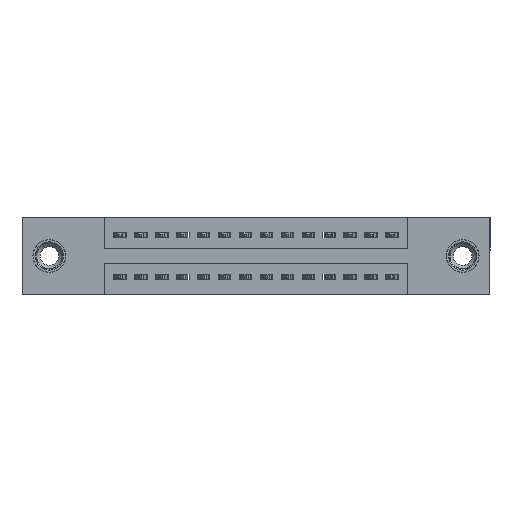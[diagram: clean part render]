
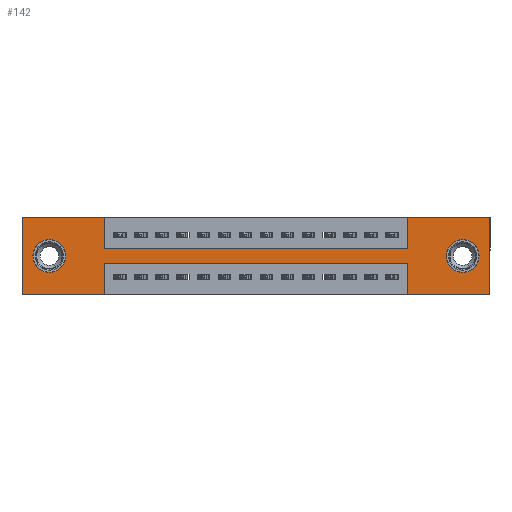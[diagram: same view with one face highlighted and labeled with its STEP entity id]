
A CAD part, front view. The second image highlights one B-rep face of the part: STEP entity #142.
In plain terms, the highlighted planar face has unit normal (0, -1, 0).
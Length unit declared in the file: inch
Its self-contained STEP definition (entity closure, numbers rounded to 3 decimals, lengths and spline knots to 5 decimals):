
#63 = VECTOR ( 'NONE', #2689, 39.37008 ) ;
#142 = ADVANCED_FACE ( 'NONE', ( #17013, #1408, #9060 ), #14671, .T. ) ;
#169 = VERTEX_POINT ( 'NONE', #14164 ) ;
#590 = CIRCLE ( 'NONE', #18414, 0.078 ) ;
#950 = CARTESIAN_POINT ( 'NONE',  ( 2.235, 0., 0. ) ) ;
#978 = CARTESIAN_POINT ( 'NONE',  ( 1.8425, 0., 0. ) ) ;
#983 = VERTEX_POINT ( 'NONE', #18829 ) ;
#1070 = CIRCLE ( 'NONE', #3841, 0.078 ) ;
#1088 = ORIENTED_EDGE ( 'NONE', *, *, #15698, .F. ) ;
#1398 = CARTESIAN_POINT ( 'NONE',  ( 2.105, 0., -0.107 ) ) ;
#1408 = FACE_BOUND ( 'NONE', #16963, .T. ) ;
#1886 = DIRECTION ( 'NONE',  ( 0., 0., -1. ) ) ;
#2145 = EDGE_CURVE ( 'NONE', #16153, #7513, #15894, .T. ) ;
#2438 = DIRECTION ( 'NONE',  ( 1., 0., 0. ) ) ;
#2542 = CARTESIAN_POINT ( 'NONE',  ( 2.105, 0., -0.185 ) ) ;
#2689 = DIRECTION ( 'NONE',  ( -1., 0., 0. ) ) ;
#2697 = VERTEX_POINT ( 'NONE', #13400 ) ;
#2744 = ORIENTED_EDGE ( 'NONE', *, *, #16561, .F. ) ;
#2795 = ORIENTED_EDGE ( 'NONE', *, *, #18884, .T. ) ;
#2824 = LINE ( 'NONE', #17985, #13924 ) ;
#2938 = EDGE_CURVE ( 'NONE', #16693, #10378, #7676, .T. ) ;
#3179 = ORIENTED_EDGE ( 'NONE', *, *, #10170, .F. ) ;
#3204 = LINE ( 'NONE', #4451, #18635 ) ;
#3341 = CARTESIAN_POINT ( 'NONE',  ( 1.8425, 0., -0.37 ) ) ;
#3640 = VECTOR ( 'NONE', #6353, 39.37008 ) ;
#3841 = AXIS2_PLACEMENT_3D ( 'NONE', #2542, #13101, #4074 ) ;
#3911 = CARTESIAN_POINT ( 'NONE',  ( 0.3925, 0., -0.15 ) ) ;
#4001 = ORIENTED_EDGE ( 'NONE', *, *, #4603, .T. ) ;
#4074 = DIRECTION ( 'NONE',  ( 0., 0., -1. ) ) ;
#4122 = LINE ( 'NONE', #4851, #3640 ) ;
#4193 = VERTEX_POINT ( 'NONE', #12833 ) ;
#4451 = CARTESIAN_POINT ( 'NONE',  ( 0., 0., 0. ) ) ;
#4603 = EDGE_CURVE ( 'NONE', #14933, #15991, #590, .T. ) ;
#4646 = ORIENTED_EDGE ( 'NONE', *, *, #14055, .T. ) ;
#4661 = VECTOR ( 'NONE', #6580, 39.37008 ) ;
#4756 = EDGE_CURVE ( 'NONE', #4193, #2697, #13933, .T. ) ;
#4851 = CARTESIAN_POINT ( 'NONE',  ( 0.3925, 0., -0.22 ) ) ;
#4906 = CARTESIAN_POINT ( 'NONE',  ( 1.8425, 0., -0.37 ) ) ;
#5013 = DIRECTION ( 'NONE',  ( 0., 1., 0. ) ) ;
#5074 = DIRECTION ( 'NONE',  ( 0., 0., -1. ) ) ;
#5104 = CARTESIAN_POINT ( 'NONE',  ( 0., 0., -0.37 ) ) ;
#5233 = LINE ( 'NONE', #8733, #63 ) ;
#5381 = DIRECTION ( 'NONE',  ( 0., 1., 0. ) ) ;
#5445 = DIRECTION ( 'NONE',  ( 0., 0., -1. ) ) ;
#5567 = DIRECTION ( 'NONE',  ( 0., -1., 0. ) ) ;
#5691 = EDGE_LOOP ( 'NONE', ( #10915, #8314, #1088, #6190, #3179, #18370, #19272, #2744, #16625, #10295, #11660, #17149 ) ) ;
#6025 = DIRECTION ( 'NONE',  ( 0., 0., 1. ) ) ;
#6065 = EDGE_LOOP ( 'NONE', ( #4646, #14043 ) ) ;
#6190 = ORIENTED_EDGE ( 'NONE', *, *, #13681, .F. ) ;
#6353 = DIRECTION ( 'NONE',  ( -1., 0., 0. ) ) ;
#6580 = DIRECTION ( 'NONE',  ( 1., 0., 0. ) ) ;
#6815 = LINE ( 'NONE', #7184, #17757 ) ;
#7184 = CARTESIAN_POINT ( 'NONE',  ( 2.235, 0., 0. ) ) ;
#7325 = LINE ( 'NONE', #3911, #18682 ) ;
#7513 = VERTEX_POINT ( 'NONE', #978 ) ;
#7608 = EDGE_CURVE ( 'NONE', #8847, #169, #3204, .T. ) ;
#7676 = LINE ( 'NONE', #15520, #15160 ) ;
#7690 = CARTESIAN_POINT ( 'NONE',  ( 0.3925, 0., -0.37 ) ) ;
#7723 = CARTESIAN_POINT ( 'NONE',  ( 0.13, 0., -0.185 ) ) ;
#7734 = AXIS2_PLACEMENT_3D ( 'NONE', #13994, #5013, #15518 ) ;
#7795 = CARTESIAN_POINT ( 'NONE',  ( 1.8425, 0., -0.15 ) ) ;
#7839 = EDGE_CURVE ( 'NONE', #983, #9812, #19305, .T. ) ;
#8314 = ORIENTED_EDGE ( 'NONE', *, *, #11064, .F. ) ;
#8733 = CARTESIAN_POINT ( 'NONE',  ( 0., 0., -0.37 ) ) ;
#8847 = VERTEX_POINT ( 'NONE', #5104 ) ;
#9060 = FACE_OUTER_BOUND ( 'NONE', #5691, .T. ) ;
#9213 = DIRECTION ( 'NONE',  ( 0., 0., 1. ) ) ;
#9723 = AXIS2_PLACEMENT_3D ( 'NONE', #14726, #5567, #5445 ) ;
#9812 = VERTEX_POINT ( 'NONE', #1398 ) ;
#9911 = LINE ( 'NONE', #3341, #17379 ) ;
#10145 = VERTEX_POINT ( 'NONE', #950 ) ;
#10170 = EDGE_CURVE ( 'NONE', #10145, #11224, #6815, .T. ) ;
#10295 = ORIENTED_EDGE ( 'NONE', *, *, #16709, .F. ) ;
#10378 = VERTEX_POINT ( 'NONE', #7690 ) ;
#10524 = CARTESIAN_POINT ( 'NONE',  ( 1.8425, 0., -0.22 ) ) ;
#10660 = CARTESIAN_POINT ( 'NONE',  ( 0.3925, 0., -0.22 ) ) ;
#10915 = ORIENTED_EDGE ( 'NONE', *, *, #2938, .F. ) ;
#10916 = VERTEX_POINT ( 'NONE', #10524 ) ;
#11064 = EDGE_CURVE ( 'NONE', #10916, #16693, #4122, .T. ) ;
#11224 = VERTEX_POINT ( 'NONE', #11235 ) ;
#11235 = CARTESIAN_POINT ( 'NONE',  ( 2.235, 0., -0.37 ) ) ;
#11535 = VERTEX_POINT ( 'NONE', #4906 ) ;
#11660 = ORIENTED_EDGE ( 'NONE', *, *, #7608, .F. ) ;
#11736 = LINE ( 'NONE', #15546, #4661 ) ;
#12465 = VECTOR ( 'NONE', #19485, 39.37008 ) ;
#12833 = CARTESIAN_POINT ( 'NONE',  ( 0.3925, 0., 0. ) ) ;
#13101 = DIRECTION ( 'NONE',  ( 0., 1., 0. ) ) ;
#13132 = DIRECTION ( 'NONE',  ( 0., 0., 1. ) ) ;
#13385 = LINE ( 'NONE', #16664, #12465 ) ;
#13400 = CARTESIAN_POINT ( 'NONE',  ( 0.3925, 0., -0.15 ) ) ;
#13412 = CARTESIAN_POINT ( 'NONE',  ( 1.8425, 0., 0. ) ) ;
#13441 = VECTOR ( 'NONE', #5074, 39.37008 ) ;
#13556 = EDGE_CURVE ( 'NONE', #10378, #8847, #5233, .T. ) ;
#13681 = EDGE_CURVE ( 'NONE', #11224, #11535, #2824, .T. ) ;
#13924 = VECTOR ( 'NONE', #15007, 39.37008 ) ;
#13933 = LINE ( 'NONE', #15586, #13441 ) ;
#13994 = CARTESIAN_POINT ( 'NONE',  ( 2.105, 0., -0.185 ) ) ;
#14043 = ORIENTED_EDGE ( 'NONE', *, *, #7839, .T. ) ;
#14055 = EDGE_CURVE ( 'NONE', #9812, #983, #1070, .T. ) ;
#14164 = CARTESIAN_POINT ( 'NONE',  ( 0., 0., 0. ) ) ;
#14353 = CARTESIAN_POINT ( 'NONE',  ( 0.13, 0., -0.185 ) ) ;
#14625 = DIRECTION ( 'NONE',  ( 0., 0., -1. ) ) ;
#14671 = PLANE ( 'NONE',  #9723 ) ;
#14726 = CARTESIAN_POINT ( 'NONE',  ( 0., 0., -0.37 ) ) ;
#14857 = CARTESIAN_POINT ( 'NONE',  ( 0.13, 0., -0.263 ) ) ;
#14933 = VERTEX_POINT ( 'NONE', #16523 ) ;
#15007 = DIRECTION ( 'NONE',  ( -1., 0., 0. ) ) ;
#15160 = VECTOR ( 'NONE', #1886, 39.37008 ) ;
#15401 = AXIS2_PLACEMENT_3D ( 'NONE', #14353, #5381, #15864 ) ;
#15518 = DIRECTION ( 'NONE',  ( 0., 0., -1. ) ) ;
#15520 = CARTESIAN_POINT ( 'NONE',  ( 0.3925, 0., -0.37 ) ) ;
#15546 = CARTESIAN_POINT ( 'NONE',  ( 0., 0., 0. ) ) ;
#15586 = CARTESIAN_POINT ( 'NONE',  ( 0.3925, 0., 0. ) ) ;
#15698 = EDGE_CURVE ( 'NONE', #11535, #10916, #9911, .T. ) ;
#15864 = DIRECTION ( 'NONE',  ( 0., 0., 1. ) ) ;
#15894 = LINE ( 'NONE', #13412, #18827 ) ;
#15991 = VERTEX_POINT ( 'NONE', #14857 ) ;
#16153 = VERTEX_POINT ( 'NONE', #7795 ) ;
#16523 = CARTESIAN_POINT ( 'NONE',  ( 0.13, 0., -0.107 ) ) ;
#16561 = EDGE_CURVE ( 'NONE', #2697, #16153, #7325, .T. ) ;
#16625 = ORIENTED_EDGE ( 'NONE', *, *, #4756, .F. ) ;
#16664 = CARTESIAN_POINT ( 'NONE',  ( 0., 0., 0. ) ) ;
#16693 = VERTEX_POINT ( 'NONE', #10660 ) ;
#16709 = EDGE_CURVE ( 'NONE', #169, #4193, #13385, .T. ) ;
#16963 = EDGE_LOOP ( 'NONE', ( #4001, #2795 ) ) ;
#17013 = FACE_BOUND ( 'NONE', #6065, .T. ) ;
#17149 = ORIENTED_EDGE ( 'NONE', *, *, #13556, .F. ) ;
#17379 = VECTOR ( 'NONE', #18585, 39.37008 ) ;
#17419 = EDGE_CURVE ( 'NONE', #7513, #10145, #11736, .T. ) ;
#17757 = VECTOR ( 'NONE', #14625, 39.37008 ) ;
#17985 = CARTESIAN_POINT ( 'NONE',  ( 0., 0., -0.37 ) ) ;
#18133 = DIRECTION ( 'NONE',  ( 0., 1., 0. ) ) ;
#18370 = ORIENTED_EDGE ( 'NONE', *, *, #17419, .F. ) ;
#18414 = AXIS2_PLACEMENT_3D ( 'NONE', #7723, #18133, #9213 ) ;
#18585 = DIRECTION ( 'NONE',  ( 0., 0., 1. ) ) ;
#18635 = VECTOR ( 'NONE', #6025, 39.37008 ) ;
#18682 = VECTOR ( 'NONE', #2438, 39.37008 ) ;
#18827 = VECTOR ( 'NONE', #13132, 39.37008 ) ;
#18829 = CARTESIAN_POINT ( 'NONE',  ( 2.105, 0., -0.263 ) ) ;
#18884 = EDGE_CURVE ( 'NONE', #15991, #14933, #19264, .T. ) ;
#19264 = CIRCLE ( 'NONE', #15401, 0.078 ) ;
#19272 = ORIENTED_EDGE ( 'NONE', *, *, #2145, .F. ) ;
#19305 = CIRCLE ( 'NONE', #7734, 0.078 ) ;
#19485 = DIRECTION ( 'NONE',  ( 1., 0., 0. ) ) ;
